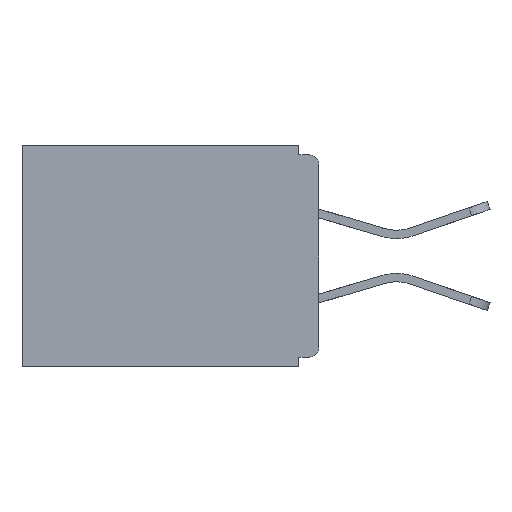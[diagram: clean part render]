
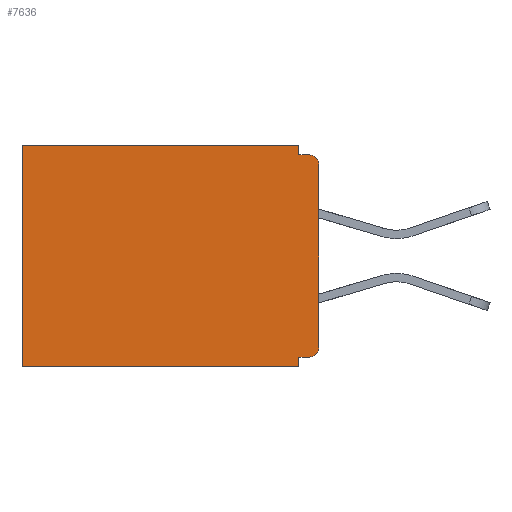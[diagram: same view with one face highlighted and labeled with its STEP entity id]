
A CAD part, left-side view. The second image highlights one B-rep face of the part: STEP entity #7636.
In plain terms, the highlighted planar face has unit normal (-1, 0, 0).
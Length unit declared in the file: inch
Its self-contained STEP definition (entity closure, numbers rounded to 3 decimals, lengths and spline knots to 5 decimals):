
#41 = EDGE_CURVE ( 'NONE', #7945, #10557, #6900, .T. ) ;
#106 = AXIS2_PLACEMENT_3D ( 'NONE', #3545, #1409, #8065 ) ;
#268 = EDGE_CURVE ( 'NONE', #7945, #12466, #10464, .T. ) ;
#451 = CARTESIAN_POINT ( 'NONE',  ( 0.298, 0., -0.313 ) ) ;
#474 = ORIENTED_EDGE ( 'NONE', *, *, #4348, .F. ) ;
#545 = EDGE_CURVE ( 'NONE', #1261, #12466, #12839, .T. ) ;
#717 = EDGE_CURVE ( 'NONE', #8134, #4017, #4134, .T. ) ;
#1114 = EDGE_LOOP ( 'NONE', ( #5613, #474, #8880, #5415, #4948, #4106, #13562, #6694, #11522, #9629 ) ) ;
#1261 = VERTEX_POINT ( 'NONE', #10416 ) ;
#1274 = VERTEX_POINT ( 'NONE', #1802 ) ;
#1328 = CARTESIAN_POINT ( 'NONE',  ( 0.298, 0.031, -0.328 ) ) ;
#1409 = DIRECTION ( 'NONE',  ( 1., 0., 0. ) ) ;
#1617 = LINE ( 'NONE', #6721, #8622 ) ;
#1802 = CARTESIAN_POINT ( 'NONE',  ( 0.298, 0.031, 0. ) ) ;
#2067 = LINE ( 'NONE', #5815, #5672 ) ;
#2830 = CARTESIAN_POINT ( 'NONE',  ( 0.298, 0.015, -0.015 ) ) ;
#3545 = CARTESIAN_POINT ( 'NONE',  ( 0.298, 0., 0. ) ) ;
#3735 = EDGE_CURVE ( 'NONE', #7370, #4017, #4193, .T. ) ;
#3804 = VECTOR ( 'NONE', #9567, 39.37008 ) ;
#4017 = VERTEX_POINT ( 'NONE', #7539 ) ;
#4106 = ORIENTED_EDGE ( 'NONE', *, *, #3735, .F. ) ;
#4134 = LINE ( 'NONE', #4184, #9946 ) ;
#4184 = CARTESIAN_POINT ( 'NONE',  ( 0.298, 0.46, 0. ) ) ;
#4193 = LINE ( 'NONE', #5995, #4698 ) ;
#4196 = VERTEX_POINT ( 'NONE', #2830 ) ;
#4348 = EDGE_CURVE ( 'NONE', #8991, #4196, #1617, .T. ) ;
#4357 = CARTESIAN_POINT ( 'NONE',  ( 0.298, 0.015, -0.328 ) ) ;
#4534 = DIRECTION ( 'NONE',  ( 0., 0., -1. ) ) ;
#4698 = VECTOR ( 'NONE', #8183, 39.37008 ) ;
#4705 = DIRECTION ( 'NONE',  ( 0., 0., -1. ) ) ;
#4948 = ORIENTED_EDGE ( 'NONE', *, *, #717, .T. ) ;
#5415 = ORIENTED_EDGE ( 'NONE', *, *, #11201, .T. ) ;
#5505 = DIRECTION ( 'NONE',  ( -1., 0., 0. ) ) ;
#5613 = ORIENTED_EDGE ( 'NONE', *, *, #6663, .T. ) ;
#5625 = VECTOR ( 'NONE', #4705, 39.37008 ) ;
#5672 = VECTOR ( 'NONE', #11229, 39.37008 ) ;
#5815 = CARTESIAN_POINT ( 'NONE',  ( 0.298, 0., 0. ) ) ;
#5995 = CARTESIAN_POINT ( 'NONE',  ( 0.298, 0., -0.343 ) ) ;
#6198 = CARTESIAN_POINT ( 'NONE',  ( 0.298, 0., -0.328 ) ) ;
#6533 = CIRCLE ( 'NONE', #7055, 0.015 ) ;
#6663 = EDGE_CURVE ( 'NONE', #1261, #4196, #6533, .T. ) ;
#6694 = ORIENTED_EDGE ( 'NONE', *, *, #41, .F. ) ;
#6721 = CARTESIAN_POINT ( 'NONE',  ( 0.298, 0., -0.015 ) ) ;
#6723 = LINE ( 'NONE', #8560, #3804 ) ;
#6900 = LINE ( 'NONE', #6198, #8607 ) ;
#7055 = AXIS2_PLACEMENT_3D ( 'NONE', #13712, #13819, #13865 ) ;
#7370 = VERTEX_POINT ( 'NONE', #8464 ) ;
#7539 = CARTESIAN_POINT ( 'NONE',  ( 0.298, 0.46, -0.343 ) ) ;
#7636 = ADVANCED_FACE ( 'NONE', ( #13079 ), #11234, .F. ) ;
#7945 = VERTEX_POINT ( 'NONE', #4357 ) ;
#8065 = DIRECTION ( 'NONE',  ( 0., 0., -1. ) ) ;
#8134 = VERTEX_POINT ( 'NONE', #9155 ) ;
#8183 = DIRECTION ( 'NONE',  ( 0., 1., 0. ) ) ;
#8464 = CARTESIAN_POINT ( 'NONE',  ( 0.298, 0.031, -0.343 ) ) ;
#8560 = CARTESIAN_POINT ( 'NONE',  ( 0.298, 0.031, -0.343 ) ) ;
#8607 = VECTOR ( 'NONE', #9393, 39.37008 ) ;
#8622 = VECTOR ( 'NONE', #10009, 39.37008 ) ;
#8880 = ORIENTED_EDGE ( 'NONE', *, *, #9849, .F. ) ;
#8991 = VERTEX_POINT ( 'NONE', #13814 ) ;
#9155 = CARTESIAN_POINT ( 'NONE',  ( 0.298, 0.46, 0. ) ) ;
#9231 = DIRECTION ( 'NONE',  ( 0., 0., -1. ) ) ;
#9380 = AXIS2_PLACEMENT_3D ( 'NONE', #12195, #5505, #4534 ) ;
#9393 = DIRECTION ( 'NONE',  ( 0., 1., 0. ) ) ;
#9567 = DIRECTION ( 'NONE',  ( 0., 0., -1. ) ) ;
#9629 = ORIENTED_EDGE ( 'NONE', *, *, #545, .F. ) ;
#9849 = EDGE_CURVE ( 'NONE', #1274, #8991, #6723, .T. ) ;
#9946 = VECTOR ( 'NONE', #13866, 39.37008 ) ;
#10009 = DIRECTION ( 'NONE',  ( 0., -1., 0. ) ) ;
#10416 = CARTESIAN_POINT ( 'NONE',  ( 0.298, 0., -0.03 ) ) ;
#10464 = CIRCLE ( 'NONE', #9380, 0.015 ) ;
#10557 = VERTEX_POINT ( 'NONE', #1328 ) ;
#10784 = VECTOR ( 'NONE', #9231, 39.37008 ) ;
#11201 = EDGE_CURVE ( 'NONE', #1274, #8134, #2067, .T. ) ;
#11229 = DIRECTION ( 'NONE',  ( 0., 1., 0. ) ) ;
#11234 = PLANE ( 'NONE',  #106 ) ;
#11522 = ORIENTED_EDGE ( 'NONE', *, *, #268, .T. ) ;
#11589 = CARTESIAN_POINT ( 'NONE',  ( 0.298, 0., 0. ) ) ;
#12195 = CARTESIAN_POINT ( 'NONE',  ( 0.298, 0.015, -0.313 ) ) ;
#12466 = VERTEX_POINT ( 'NONE', #451 ) ;
#12839 = LINE ( 'NONE', #11589, #10784 ) ;
#13079 = FACE_OUTER_BOUND ( 'NONE', #1114, .T. ) ;
#13264 = CARTESIAN_POINT ( 'NONE',  ( 0.298, 0.031, -0.343 ) ) ;
#13290 = EDGE_CURVE ( 'NONE', #10557, #7370, #14113, .T. ) ;
#13562 = ORIENTED_EDGE ( 'NONE', *, *, #13290, .F. ) ;
#13712 = CARTESIAN_POINT ( 'NONE',  ( 0.298, 0.015, -0.03 ) ) ;
#13814 = CARTESIAN_POINT ( 'NONE',  ( 0.298, 0.031, -0.015 ) ) ;
#13819 = DIRECTION ( 'NONE',  ( -1., 0., 0. ) ) ;
#13865 = DIRECTION ( 'NONE',  ( 0., 0., -1. ) ) ;
#13866 = DIRECTION ( 'NONE',  ( 0., 0., -1. ) ) ;
#14113 = LINE ( 'NONE', #13264, #5625 ) ;
